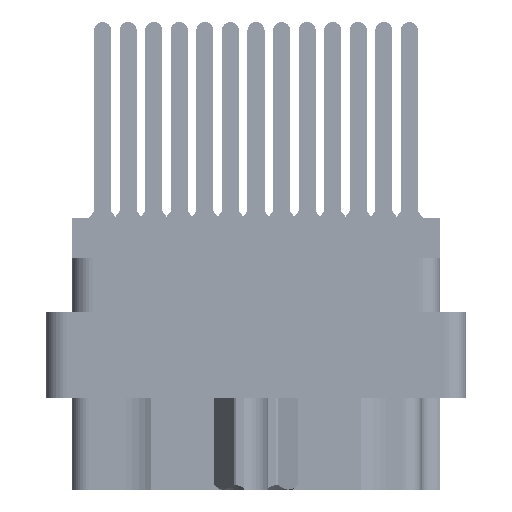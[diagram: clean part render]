
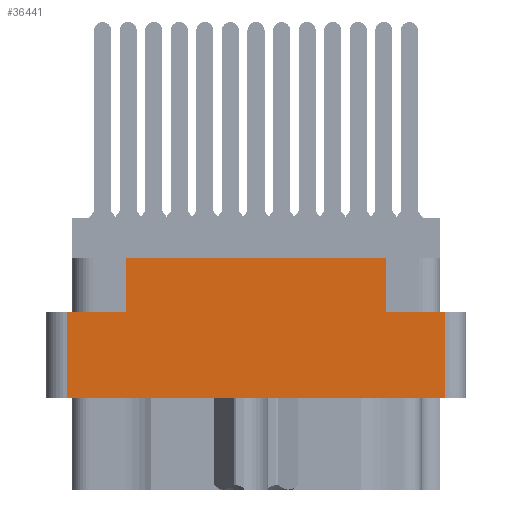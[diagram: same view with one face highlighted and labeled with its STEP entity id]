
A CAD part, left-side view. The second image highlights one B-rep face of the part: STEP entity #36441.
In plain terms, the highlighted planar face has unit normal (-1, 0, 0).
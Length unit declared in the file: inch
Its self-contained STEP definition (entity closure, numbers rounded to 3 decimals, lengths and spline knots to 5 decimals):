
#2069 = LINE ( 'NONE', #44424, #68796 ) ;
#2928 = DIRECTION ( 'NONE',  ( -1., 0., 0. ) ) ;
#3014 = EDGE_CURVE ( 'NONE', #35058, #36518, #16307, .T. ) ;
#3944 = LINE ( 'NONE', #52241, #33379 ) ;
#6329 = CARTESIAN_POINT ( 'NONE',  ( -1.359, -0.3825, -0.277 ) ) ;
#6801 = VECTOR ( 'NONE', #7348, 39.37008 ) ;
#6916 = CARTESIAN_POINT ( 'NONE',  ( -1.359, -0.3825, -0.117 ) ) ;
#7348 = DIRECTION ( 'NONE',  ( 0., 0., 1. ) ) ;
#13660 = EDGE_CURVE ( 'NONE', #58220, #36518, #3944, .T. ) ;
#14925 = VERTEX_POINT ( 'NONE', #21803 ) ;
#16307 = LINE ( 'NONE', #72955, #65895 ) ;
#16662 = ORIENTED_EDGE ( 'NONE', *, *, #32785, .F. ) ;
#19233 = ORIENTED_EDGE ( 'NONE', *, *, #13660, .F. ) ;
#19817 = AXIS2_PLACEMENT_3D ( 'NONE', #67343, #2928, #48983 ) ;
#20840 = CARTESIAN_POINT ( 'NONE',  ( -1.359, 0., -0.277 ) ) ;
#21803 = CARTESIAN_POINT ( 'NONE',  ( -1.359, -0.555, -0.277 ) ) ;
#22995 = CARTESIAN_POINT ( 'NONE',  ( -1.359, 0.555, -0.529 ) ) ;
#24230 = VECTOR ( 'NONE', #41753, 39.37008 ) ;
#24747 = VECTOR ( 'NONE', #27380, 39.37008 ) ;
#27380 = DIRECTION ( 'NONE',  ( 0., -1., 0. ) ) ;
#29102 = EDGE_CURVE ( 'NONE', #35058, #60816, #37944, .T. ) ;
#29862 = FACE_OUTER_BOUND ( 'NONE', #53580, .T. ) ;
#30242 = ORIENTED_EDGE ( 'NONE', *, *, #51422, .T. ) ;
#30830 = DIRECTION ( 'NONE',  ( 0., -1., 0. ) ) ;
#30906 = CARTESIAN_POINT ( 'NONE',  ( -1.359, 0.3825, -0.117 ) ) ;
#31586 = CARTESIAN_POINT ( 'NONE',  ( -1.359, -0.555, -0.529 ) ) ;
#32785 = EDGE_CURVE ( 'NONE', #82426, #58314, #2069, .T. ) ;
#33321 = DIRECTION ( 'NONE',  ( 0., 0., 1. ) ) ;
#33379 = VECTOR ( 'NONE', #65753, 39.37008 ) ;
#33495 = DIRECTION ( 'NONE',  ( 0., 0., -1. ) ) ;
#35058 = VERTEX_POINT ( 'NONE', #37953 ) ;
#36441 = ADVANCED_FACE ( 'NONE', ( #29862 ), #41701, .T. ) ;
#36518 = VERTEX_POINT ( 'NONE', #22995 ) ;
#37944 = LINE ( 'NONE', #20840, #24747 ) ;
#37953 = CARTESIAN_POINT ( 'NONE',  ( -1.359, 0.555, -0.277 ) ) ;
#41701 = PLANE ( 'NONE',  #19817 ) ;
#41753 = DIRECTION ( 'NONE',  ( 0., 0., 1. ) ) ;
#42741 = ORIENTED_EDGE ( 'NONE', *, *, #3014, .T. ) ;
#44424 = CARTESIAN_POINT ( 'NONE',  ( -1.359, 0.617, -0.117 ) ) ;
#46353 = ORIENTED_EDGE ( 'NONE', *, *, #75537, .F. ) ;
#48136 = ORIENTED_EDGE ( 'NONE', *, *, #29102, .F. ) ;
#48983 = DIRECTION ( 'NONE',  ( 0., 0., 1. ) ) ;
#49643 = LINE ( 'NONE', #68237, #24230 ) ;
#51422 = EDGE_CURVE ( 'NONE', #69708, #58314, #69491, .T. ) ;
#52241 = CARTESIAN_POINT ( 'NONE',  ( -1.359, 0., -0.529 ) ) ;
#52417 = ORIENTED_EDGE ( 'NONE', *, *, #79925, .T. ) ;
#53580 = EDGE_LOOP ( 'NONE', ( #48136, #42741, #19233, #52417, #46353, #30242, #16662, #79764 ) ) ;
#57416 = DIRECTION ( 'NONE',  ( 0., -1., 0. ) ) ;
#58220 = VERTEX_POINT ( 'NONE', #31586 ) ;
#58314 = VERTEX_POINT ( 'NONE', #6916 ) ;
#60816 = VERTEX_POINT ( 'NONE', #83095 ) ;
#65753 = DIRECTION ( 'NONE',  ( 0., 1., 0. ) ) ;
#65895 = VECTOR ( 'NONE', #33495, 39.37008 ) ;
#67343 = CARTESIAN_POINT ( 'NONE',  ( -1.359, -0.617, -0.798 ) ) ;
#68237 = CARTESIAN_POINT ( 'NONE',  ( -1.359, -0.555, -0.798 ) ) ;
#68796 = VECTOR ( 'NONE', #57416, 39.37008 ) ;
#69481 = CARTESIAN_POINT ( 'NONE',  ( -1.359, 0., -0.277 ) ) ;
#69491 = LINE ( 'NONE', #78201, #6801 ) ;
#69708 = VERTEX_POINT ( 'NONE', #6329 ) ;
#71379 = CARTESIAN_POINT ( 'NONE',  ( -1.359, 0.3825, -0.277 ) ) ;
#72955 = CARTESIAN_POINT ( 'NONE',  ( -1.359, 0.555, -0.798 ) ) ;
#74156 = LINE ( 'NONE', #69481, #79216 ) ;
#74778 = LINE ( 'NONE', #71379, #77730 ) ;
#75537 = EDGE_CURVE ( 'NONE', #69708, #14925, #74156, .T. ) ;
#77730 = VECTOR ( 'NONE', #33321, 39.37008 ) ;
#78201 = CARTESIAN_POINT ( 'NONE',  ( -1.359, -0.3825, -0.277 ) ) ;
#79216 = VECTOR ( 'NONE', #30830, 39.37008 ) ;
#79552 = EDGE_CURVE ( 'NONE', #60816, #82426, #74778, .T. ) ;
#79764 = ORIENTED_EDGE ( 'NONE', *, *, #79552, .F. ) ;
#79925 = EDGE_CURVE ( 'NONE', #58220, #14925, #49643, .T. ) ;
#82426 = VERTEX_POINT ( 'NONE', #30906 ) ;
#83095 = CARTESIAN_POINT ( 'NONE',  ( -1.359, 0.3825, -0.277 ) ) ;
